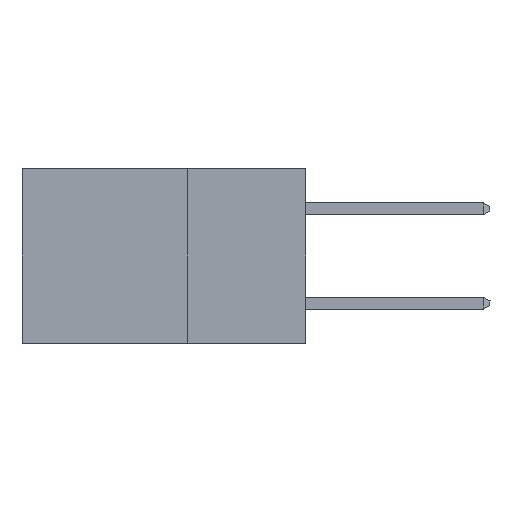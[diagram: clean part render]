
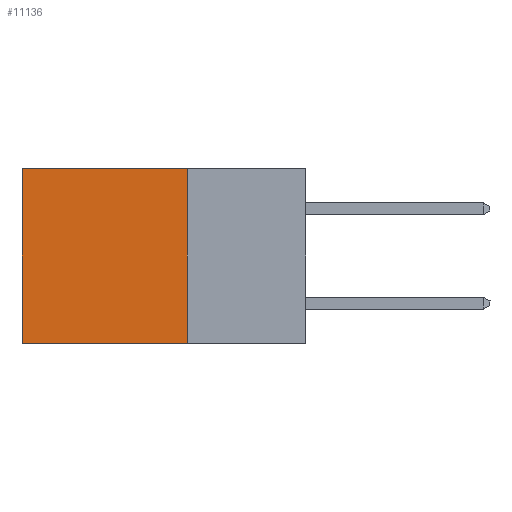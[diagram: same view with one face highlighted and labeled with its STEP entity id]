
A CAD part, left-side view. The second image highlights one B-rep face of the part: STEP entity #11136.
In plain terms, the highlighted planar face has unit normal (-1, 0, 0).
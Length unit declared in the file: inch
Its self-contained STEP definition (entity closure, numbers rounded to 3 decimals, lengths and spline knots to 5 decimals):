
#1072 = DIRECTION ( 'NONE',  ( 0., 1., 0. ) ) ;
#1591 = VERTEX_POINT ( 'NONE', #14005 ) ;
#1895 = VECTOR ( 'NONE', #5372, 39.37008 ) ;
#2030 = PLANE ( 'NONE',  #23899 ) ;
#2902 = VECTOR ( 'NONE', #25073, 39.37008 ) ;
#3707 = CARTESIAN_POINT ( 'NONE',  ( 0.298, 0.25, 0. ) ) ;
#3808 = EDGE_CURVE ( 'NONE', #13040, #1591, #23317, .T. ) ;
#5271 = LINE ( 'NONE', #17993, #6010 ) ;
#5372 = DIRECTION ( 'NONE',  ( 0., 1., 0. ) ) ;
#5904 = VERTEX_POINT ( 'NONE', #9797 ) ;
#6010 = VECTOR ( 'NONE', #11070, 39.37008 ) ;
#7633 = CARTESIAN_POINT ( 'NONE',  ( 0.298, 0.25, 0. ) ) ;
#7800 = EDGE_LOOP ( 'NONE', ( #19298, #9941, #25321, #10835 ) ) ;
#8098 = FACE_OUTER_BOUND ( 'NONE', #7800, .T. ) ;
#9013 = EDGE_CURVE ( 'NONE', #16262, #5904, #5271, .T. ) ;
#9797 = CARTESIAN_POINT ( 'NONE',  ( 0.298, 0.6, -0.37 ) ) ;
#9941 = ORIENTED_EDGE ( 'NONE', *, *, #18901, .F. ) ;
#10835 = ORIENTED_EDGE ( 'NONE', *, *, #18494, .T. ) ;
#11070 = DIRECTION ( 'NONE',  ( 0., 0., -1. ) ) ;
#11136 = ADVANCED_FACE ( 'NONE', ( #8098 ), #2030, .F. ) ;
#13040 = VERTEX_POINT ( 'NONE', #13106 ) ;
#13106 = CARTESIAN_POINT ( 'NONE',  ( 0.298, 0.25, 0. ) ) ;
#14005 = CARTESIAN_POINT ( 'NONE',  ( 0.298, 0.25, -0.37 ) ) ;
#16262 = VERTEX_POINT ( 'NONE', #18929 ) ;
#17993 = CARTESIAN_POINT ( 'NONE',  ( 0.298, 0.6, 0. ) ) ;
#18494 = EDGE_CURVE ( 'NONE', #13040, #16262, #28595, .T. ) ;
#18516 = CARTESIAN_POINT ( 'NONE',  ( 0.298, 0.25, 0. ) ) ;
#18831 = DIRECTION ( 'NONE',  ( 0., 0., -1. ) ) ;
#18901 = EDGE_CURVE ( 'NONE', #1591, #5904, #28191, .T. ) ;
#18929 = CARTESIAN_POINT ( 'NONE',  ( 0.298, 0.6, 0. ) ) ;
#19298 = ORIENTED_EDGE ( 'NONE', *, *, #9013, .T. ) ;
#22237 = CARTESIAN_POINT ( 'NONE',  ( 0.298, 0.25, -0.37 ) ) ;
#23317 = LINE ( 'NONE', #3707, #2902 ) ;
#23899 = AXIS2_PLACEMENT_3D ( 'NONE', #18516, #30487, #18831 ) ;
#25073 = DIRECTION ( 'NONE',  ( 0., 0., -1. ) ) ;
#25321 = ORIENTED_EDGE ( 'NONE', *, *, #3808, .F. ) ;
#26742 = VECTOR ( 'NONE', #1072, 39.37008 ) ;
#28191 = LINE ( 'NONE', #22237, #26742 ) ;
#28595 = LINE ( 'NONE', #7633, #1895 ) ;
#30487 = DIRECTION ( 'NONE',  ( 1., 0., 0. ) ) ;
